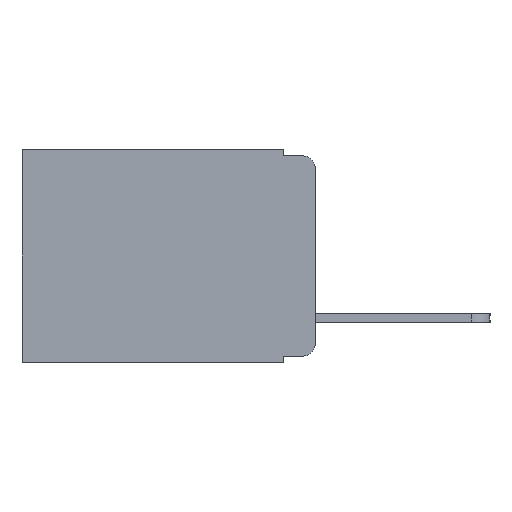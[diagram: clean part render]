
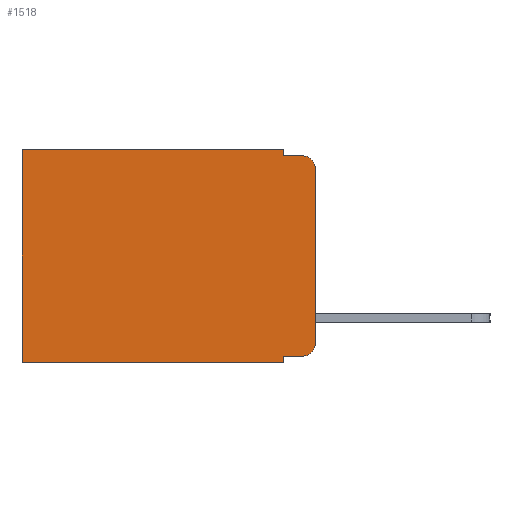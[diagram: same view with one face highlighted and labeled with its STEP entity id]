
A CAD part, left-side view. The second image highlights one B-rep face of the part: STEP entity #1518.
In plain terms, the highlighted planar face has unit normal (-1, 0, 0).
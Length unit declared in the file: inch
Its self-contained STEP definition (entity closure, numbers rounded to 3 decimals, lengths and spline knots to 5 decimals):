
#172 = ORIENTED_EDGE ( 'NONE', *, *, #6765, .F. ) ;
#291 = ORIENTED_EDGE ( 'NONE', *, *, #10159, .T. ) ;
#394 = CARTESIAN_POINT ( 'NONE',  ( 0.298, 0., -0.03 ) ) ;
#500 = CARTESIAN_POINT ( 'NONE',  ( 0.298, 0.051, -0.333 ) ) ;
#798 = CARTESIAN_POINT ( 'NONE',  ( 0.298, 0., -0.343 ) ) ;
#871 = DIRECTION ( 'NONE',  ( 0., 1., 0. ) ) ;
#1050 = ORIENTED_EDGE ( 'NONE', *, *, #4988, .T. ) ;
#1384 = DIRECTION ( 'NONE',  ( 1., 0., 0. ) ) ;
#1479 = AXIS2_PLACEMENT_3D ( 'NONE', #8094, #2941, #8945 ) ;
#1518 = ADVANCED_FACE ( 'NONE', ( #8365 ), #10717, .F. ) ;
#1565 = AXIS2_PLACEMENT_3D ( 'NONE', #3903, #1384, #4046 ) ;
#1785 = ORIENTED_EDGE ( 'NONE', *, *, #9242, .T. ) ;
#2052 = CARTESIAN_POINT ( 'NONE',  ( 0.298, 0., -0.313 ) ) ;
#2238 = VECTOR ( 'NONE', #2767, 39.37008 ) ;
#2289 = ORIENTED_EDGE ( 'NONE', *, *, #2731, .F. ) ;
#2356 = VECTOR ( 'NONE', #871, 39.37008 ) ;
#2412 = CIRCLE ( 'NONE', #1479, 0.02 ) ;
#2460 = VERTEX_POINT ( 'NONE', #3573 ) ;
#2590 = CARTESIAN_POINT ( 'NONE',  ( 0.298, 0.473, 0. ) ) ;
#2731 = EDGE_CURVE ( 'NONE', #9855, #3438, #5798, .T. ) ;
#2767 = DIRECTION ( 'NONE',  ( 0., 0., -1. ) ) ;
#2806 = CARTESIAN_POINT ( 'NONE',  ( 0.298, 0.051, 0. ) ) ;
#2820 = CARTESIAN_POINT ( 'NONE',  ( 0.298, 0.473, -0.343 ) ) ;
#2941 = DIRECTION ( 'NONE',  ( -1., 0., 0. ) ) ;
#3182 = DIRECTION ( 'NONE',  ( 0., -1., 0. ) ) ;
#3319 = VECTOR ( 'NONE', #3853, 39.37008 ) ;
#3438 = VERTEX_POINT ( 'NONE', #8013 ) ;
#3532 = VERTEX_POINT ( 'NONE', #9606 ) ;
#3573 = CARTESIAN_POINT ( 'NONE',  ( 0.298, 0.051, -0.333 ) ) ;
#3614 = ORIENTED_EDGE ( 'NONE', *, *, #6405, .F. ) ;
#3683 = VERTEX_POINT ( 'NONE', #2052 ) ;
#3696 = VERTEX_POINT ( 'NONE', #7146 ) ;
#3781 = VECTOR ( 'NONE', #4559, 39.37008 ) ;
#3853 = DIRECTION ( 'NONE',  ( 0., 0., -1. ) ) ;
#3903 = CARTESIAN_POINT ( 'NONE',  ( 0.298, 0., 0. ) ) ;
#3989 = CARTESIAN_POINT ( 'NONE',  ( 0.298, 0., 0. ) ) ;
#4046 = DIRECTION ( 'NONE',  ( 0., 0., -1. ) ) ;
#4304 = LINE ( 'NONE', #8341, #8856 ) ;
#4555 = LINE ( 'NONE', #2806, #2238 ) ;
#4559 = DIRECTION ( 'NONE',  ( 0., 1., 0. ) ) ;
#4988 = EDGE_CURVE ( 'NONE', #6122, #3683, #6835, .T. ) ;
#5163 = ORIENTED_EDGE ( 'NONE', *, *, #10084, .T. ) ;
#5778 = ORIENTED_EDGE ( 'NONE', *, *, #6516, .F. ) ;
#5782 = EDGE_CURVE ( 'NONE', #9257, #6888, #9486, .T. ) ;
#5798 = LINE ( 'NONE', #6139, #8075 ) ;
#5866 = DIRECTION ( 'NONE',  ( 0., 0., -1. ) ) ;
#6122 = VERTEX_POINT ( 'NONE', #8161 ) ;
#6139 = CARTESIAN_POINT ( 'NONE',  ( 0.298, 0.051, 0. ) ) ;
#6382 = DIRECTION ( 'NONE',  ( 0., 0., -1. ) ) ;
#6405 = EDGE_CURVE ( 'NONE', #7439, #3683, #10122, .T. ) ;
#6516 = EDGE_CURVE ( 'NONE', #2460, #3532, #4555, .T. ) ;
#6525 = AXIS2_PLACEMENT_3D ( 'NONE', #9441, #9418, #9378 ) ;
#6765 = EDGE_CURVE ( 'NONE', #3532, #6888, #8951, .T. ) ;
#6835 = CIRCLE ( 'NONE', #6525, 0.02 ) ;
#6888 = VERTEX_POINT ( 'NONE', #2820 ) ;
#7146 = CARTESIAN_POINT ( 'NONE',  ( 0.298, 0.02, -0.01 ) ) ;
#7251 = VECTOR ( 'NONE', #5866, 39.37008 ) ;
#7439 = VERTEX_POINT ( 'NONE', #394 ) ;
#7654 = ORIENTED_EDGE ( 'NONE', *, *, #5782, .T. ) ;
#7944 = CARTESIAN_POINT ( 'NONE',  ( 0.298, 0.051, 0. ) ) ;
#8013 = CARTESIAN_POINT ( 'NONE',  ( 0.298, 0.051, -0.01 ) ) ;
#8075 = VECTOR ( 'NONE', #6382, 39.37008 ) ;
#8085 = ORIENTED_EDGE ( 'NONE', *, *, #10777, .F. ) ;
#8094 = CARTESIAN_POINT ( 'NONE',  ( 0.298, 0.02, -0.03 ) ) ;
#8161 = CARTESIAN_POINT ( 'NONE',  ( 0.298, 0.02, -0.333 ) ) ;
#8212 = VECTOR ( 'NONE', #9889, 39.37008 ) ;
#8341 = CARTESIAN_POINT ( 'NONE',  ( 0.298, 0.051, -0.01 ) ) ;
#8365 = FACE_OUTER_BOUND ( 'NONE', #10413, .T. ) ;
#8475 = LINE ( 'NONE', #500, #8212 ) ;
#8847 = CARTESIAN_POINT ( 'NONE',  ( 0.298, 0.473, 0. ) ) ;
#8856 = VECTOR ( 'NONE', #3182, 39.37008 ) ;
#8945 = DIRECTION ( 'NONE',  ( 0., 0., -1. ) ) ;
#8951 = LINE ( 'NONE', #798, #2356 ) ;
#9242 = EDGE_CURVE ( 'NONE', #9855, #9257, #10550, .T. ) ;
#9257 = VERTEX_POINT ( 'NONE', #8847 ) ;
#9378 = DIRECTION ( 'NONE',  ( 0., 0., -1. ) ) ;
#9418 = DIRECTION ( 'NONE',  ( -1., 0., 0. ) ) ;
#9441 = CARTESIAN_POINT ( 'NONE',  ( 0.298, 0.02, -0.313 ) ) ;
#9486 = LINE ( 'NONE', #2590, #7251 ) ;
#9606 = CARTESIAN_POINT ( 'NONE',  ( 0.298, 0.051, -0.343 ) ) ;
#9855 = VERTEX_POINT ( 'NONE', #7944 ) ;
#9889 = DIRECTION ( 'NONE',  ( 0., -1., 0. ) ) ;
#10084 = EDGE_CURVE ( 'NONE', #7439, #3696, #2412, .T. ) ;
#10122 = LINE ( 'NONE', #3989, #3319 ) ;
#10159 = EDGE_CURVE ( 'NONE', #2460, #6122, #8475, .T. ) ;
#10413 = EDGE_LOOP ( 'NONE', ( #3614, #5163, #8085, #2289, #1785, #7654, #172, #5778, #291, #1050 ) ) ;
#10441 = CARTESIAN_POINT ( 'NONE',  ( 0.298, 0., 0. ) ) ;
#10550 = LINE ( 'NONE', #10441, #3781 ) ;
#10717 = PLANE ( 'NONE',  #1565 ) ;
#10777 = EDGE_CURVE ( 'NONE', #3438, #3696, #4304, .T. ) ;
